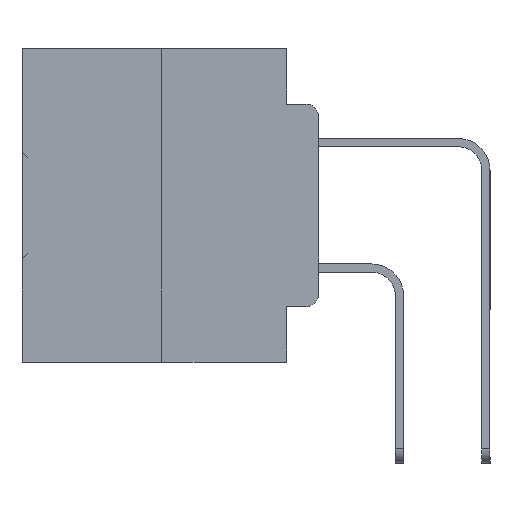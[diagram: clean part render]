
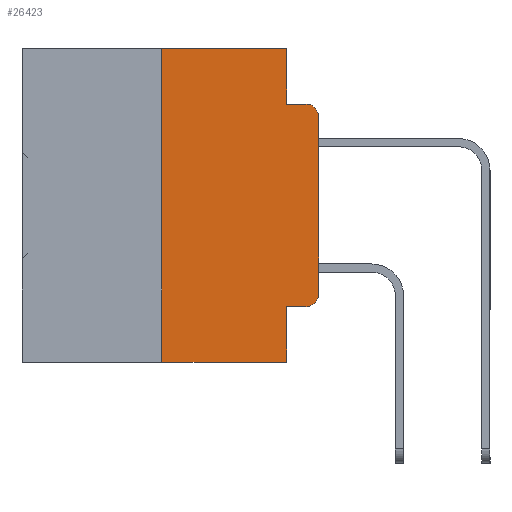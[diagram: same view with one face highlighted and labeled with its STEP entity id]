
A CAD part, left-side view. The second image highlights one B-rep face of the part: STEP entity #26423.
In plain terms, the highlighted planar face has unit normal (-1, 0, 0).
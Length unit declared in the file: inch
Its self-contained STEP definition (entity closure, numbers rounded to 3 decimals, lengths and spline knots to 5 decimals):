
#138 = DIRECTION ( 'NONE',  ( 0., -1., 0. ) ) ;
#419 = CARTESIAN_POINT ( 'NONE',  ( 0., 0.051, -0.4115 ) ) ;
#635 = CARTESIAN_POINT ( 'NONE',  ( 0., 0.25, -0.5 ) ) ;
#909 = DIRECTION ( 'NONE',  ( 0., -1., 0. ) ) ;
#2114 = CARTESIAN_POINT ( 'NONE',  ( 0., 0.25, 0. ) ) ;
#2371 = CARTESIAN_POINT ( 'NONE',  ( 0., 0., 0. ) ) ;
#2453 = CARTESIAN_POINT ( 'NONE',  ( 0., 0.051, 0. ) ) ;
#2797 = DIRECTION ( 'NONE',  ( 0., 0., -1. ) ) ;
#2968 = LINE ( 'NONE', #12059, #26030 ) ;
#3107 = VECTOR ( 'NONE', #20661, 39.37008 ) ;
#3715 = CARTESIAN_POINT ( 'NONE',  ( 0., 0.02, -0.4115 ) ) ;
#4078 = CARTESIAN_POINT ( 'NONE',  ( 0., 0.051, -0.4115 ) ) ;
#4975 = LINE ( 'NONE', #2371, #27112 ) ;
#5742 = VERTEX_POINT ( 'NONE', #12359 ) ;
#5747 = CARTESIAN_POINT ( 'NONE',  ( 0., 0., -0.3915 ) ) ;
#6008 = DIRECTION ( 'NONE',  ( -1., 0., 0. ) ) ;
#8177 = VERTEX_POINT ( 'NONE', #4078 ) ;
#8456 = ORIENTED_EDGE ( 'NONE', *, *, #11837, .F. ) ;
#9706 = LINE ( 'NONE', #2453, #34409 ) ;
#9781 = EDGE_CURVE ( 'NONE', #27792, #17400, #33629, .T. ) ;
#10172 = CARTESIAN_POINT ( 'NONE',  ( 0., 0.473, -0.5 ) ) ;
#10204 = VERTEX_POINT ( 'NONE', #22277 ) ;
#10299 = DIRECTION ( 'NONE',  ( 0., -1., 0. ) ) ;
#10721 = ORIENTED_EDGE ( 'NONE', *, *, #29102, .F. ) ;
#11078 = CARTESIAN_POINT ( 'NONE',  ( 0., 0.051, 0. ) ) ;
#11116 = CIRCLE ( 'NONE', #29280, 0.02 ) ;
#11441 = PLANE ( 'NONE',  #19000 ) ;
#11837 = EDGE_CURVE ( 'NONE', #8177, #30896, #9706, .T. ) ;
#12059 = CARTESIAN_POINT ( 'NONE',  ( 0., 0.051, 0. ) ) ;
#12358 = VERTEX_POINT ( 'NONE', #33668 ) ;
#12359 = CARTESIAN_POINT ( 'NONE',  ( 0., 0.051, -0.0885 ) ) ;
#12879 = CARTESIAN_POINT ( 'NONE',  ( 0., 0.051, -0.5 ) ) ;
#13112 = EDGE_CURVE ( 'NONE', #17400, #10204, #4975, .T. ) ;
#13550 = ORIENTED_EDGE ( 'NONE', *, *, #13112, .T. ) ;
#14478 = LINE ( 'NONE', #18279, #28848 ) ;
#15174 = LINE ( 'NONE', #2114, #37078 ) ;
#15323 = CARTESIAN_POINT ( 'NONE',  ( 0., 0.02, -0.1085 ) ) ;
#16082 = VECTOR ( 'NONE', #10299, 39.37008 ) ;
#16698 = DIRECTION ( 'NONE',  ( 0., 0., 1. ) ) ;
#17400 = VERTEX_POINT ( 'NONE', #5747 ) ;
#18224 = DIRECTION ( 'NONE',  ( 0., 0., -1. ) ) ;
#18279 = CARTESIAN_POINT ( 'NONE',  ( 0., 0.473, 0. ) ) ;
#18541 = LINE ( 'NONE', #419, #3107 ) ;
#19000 = AXIS2_PLACEMENT_3D ( 'NONE', #31554, #20118, #2797 ) ;
#19507 = ORIENTED_EDGE ( 'NONE', *, *, #28351, .F. ) ;
#20118 = DIRECTION ( 'NONE',  ( 1., 0., 0. ) ) ;
#20399 = CARTESIAN_POINT ( 'NONE',  ( 0., 0.051, -0.0885 ) ) ;
#20609 = EDGE_CURVE ( 'NONE', #5742, #12358, #21332, .T. ) ;
#20641 = ORIENTED_EDGE ( 'NONE', *, *, #25896, .T. ) ;
#20661 = DIRECTION ( 'NONE',  ( 0., -1., 0. ) ) ;
#21332 = LINE ( 'NONE', #20399, #22242 ) ;
#22242 = VECTOR ( 'NONE', #138, 39.37008 ) ;
#22265 = EDGE_LOOP ( 'NONE', ( #13550, #23478, #25373, #19507, #24937, #10721, #28691, #8456, #20641, #23341 ) ) ;
#22277 = CARTESIAN_POINT ( 'NONE',  ( 0., 0., -0.1085 ) ) ;
#22587 = DIRECTION ( 'NONE',  ( 0., 0., 1. ) ) ;
#22644 = EDGE_CURVE ( 'NONE', #26398, #28148, #14478, .T. ) ;
#22891 = CARTESIAN_POINT ( 'NONE',  ( 0., 0.25, 0. ) ) ;
#23151 = AXIS2_PLACEMENT_3D ( 'NONE', #23298, #6008, #26209 ) ;
#23298 = CARTESIAN_POINT ( 'NONE',  ( 0., 0.02, -0.3915 ) ) ;
#23341 = ORIENTED_EDGE ( 'NONE', *, *, #9781, .T. ) ;
#23478 = ORIENTED_EDGE ( 'NONE', *, *, #36768, .T. ) ;
#23706 = LINE ( 'NONE', #10172, #16082 ) ;
#24937 = ORIENTED_EDGE ( 'NONE', *, *, #22644, .F. ) ;
#25373 = ORIENTED_EDGE ( 'NONE', *, *, #20609, .F. ) ;
#25583 = DIRECTION ( 'NONE',  ( 0., 0., -1. ) ) ;
#25896 = EDGE_CURVE ( 'NONE', #8177, #27792, #18541, .T. ) ;
#26030 = VECTOR ( 'NONE', #29268, 39.37008 ) ;
#26209 = DIRECTION ( 'NONE',  ( 0., 0., -1. ) ) ;
#26398 = VERTEX_POINT ( 'NONE', #22891 ) ;
#26423 = ADVANCED_FACE ( 'NONE', ( #29738 ), #11441, .F. ) ;
#27112 = VECTOR ( 'NONE', #22587, 39.37008 ) ;
#27792 = VERTEX_POINT ( 'NONE', #3715 ) ;
#28148 = VERTEX_POINT ( 'NONE', #11078 ) ;
#28351 = EDGE_CURVE ( 'NONE', #28148, #5742, #2968, .T. ) ;
#28428 = VERTEX_POINT ( 'NONE', #635 ) ;
#28691 = ORIENTED_EDGE ( 'NONE', *, *, #33967, .T. ) ;
#28848 = VECTOR ( 'NONE', #909, 39.37008 ) ;
#29102 = EDGE_CURVE ( 'NONE', #28428, #26398, #15174, .T. ) ;
#29268 = DIRECTION ( 'NONE',  ( 0., 0., -1. ) ) ;
#29280 = AXIS2_PLACEMENT_3D ( 'NONE', #15323, #35340, #18224 ) ;
#29738 = FACE_OUTER_BOUND ( 'NONE', #22265, .T. ) ;
#30896 = VERTEX_POINT ( 'NONE', #12879 ) ;
#31554 = CARTESIAN_POINT ( 'NONE',  ( 0., 0.473, 0. ) ) ;
#33629 = CIRCLE ( 'NONE', #23151, 0.02 ) ;
#33668 = CARTESIAN_POINT ( 'NONE',  ( 0., 0.02, -0.0885 ) ) ;
#33967 = EDGE_CURVE ( 'NONE', #28428, #30896, #23706, .T. ) ;
#34409 = VECTOR ( 'NONE', #25583, 39.37008 ) ;
#35340 = DIRECTION ( 'NONE',  ( -1., 0., 0. ) ) ;
#36768 = EDGE_CURVE ( 'NONE', #10204, #12358, #11116, .T. ) ;
#37078 = VECTOR ( 'NONE', #16698, 39.37008 ) ;
